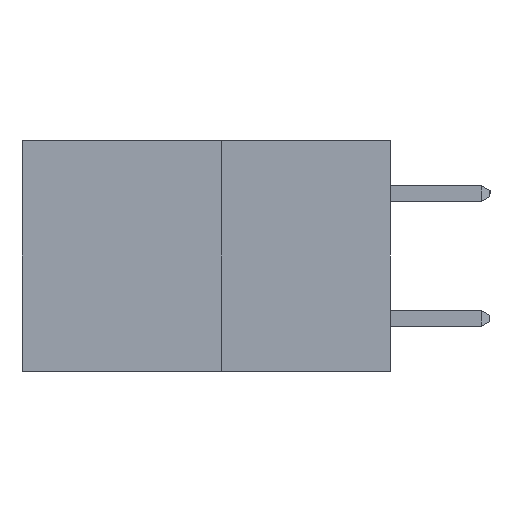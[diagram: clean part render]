
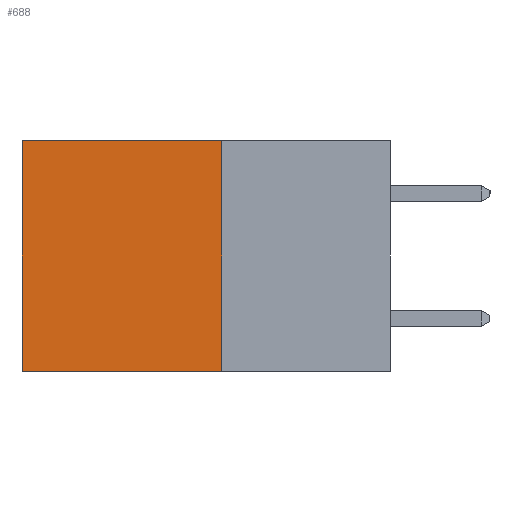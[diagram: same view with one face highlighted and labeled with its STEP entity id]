
A CAD part, left-side view. The second image highlights one B-rep face of the part: STEP entity #688.
In plain terms, the highlighted planar face has unit normal (-1, 0, 0).
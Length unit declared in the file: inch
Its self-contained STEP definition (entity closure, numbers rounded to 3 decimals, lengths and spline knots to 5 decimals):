
#74 = EDGE_CURVE ( 'NONE', #7495, #535, #5018, .T. ) ;
#273 = EDGE_LOOP ( 'NONE', ( #4200, #5590, #5253, #2440 ) ) ;
#535 = VERTEX_POINT ( 'NONE', #8804 ) ;
#688 = ADVANCED_FACE ( 'NONE', ( #9331 ), #6333, .F. ) ;
#1500 = DIRECTION ( 'NONE',  ( 1., 0., 0. ) ) ;
#1532 = VECTOR ( 'NONE', #4973, 39.37008 ) ;
#1788 = DIRECTION ( 'NONE',  ( 0., 1., 0. ) ) ;
#2301 = LINE ( 'NONE', #4025, #3783 ) ;
#2440 = ORIENTED_EDGE ( 'NONE', *, *, #3408, .T. ) ;
#2899 = VERTEX_POINT ( 'NONE', #4318 ) ;
#3270 = DIRECTION ( 'NONE',  ( 0., 0., -1. ) ) ;
#3338 = CARTESIAN_POINT ( 'NONE',  ( 0.277, 0.27, -0.37 ) ) ;
#3408 = EDGE_CURVE ( 'NONE', #4252, #2899, #2301, .T. ) ;
#3503 = LINE ( 'NONE', #4363, #1532 ) ;
#3783 = VECTOR ( 'NONE', #7253, 39.37008 ) ;
#3998 = CARTESIAN_POINT ( 'NONE',  ( 0.277, 0.27, 0. ) ) ;
#4025 = CARTESIAN_POINT ( 'NONE',  ( 0.277, 0.27, 0. ) ) ;
#4200 = ORIENTED_EDGE ( 'NONE', *, *, #6737, .T. ) ;
#4252 = VERTEX_POINT ( 'NONE', #3998 ) ;
#4318 = CARTESIAN_POINT ( 'NONE',  ( 0.277, 0.59, 0. ) ) ;
#4363 = CARTESIAN_POINT ( 'NONE',  ( 0.277, 0.59, -0.37 ) ) ;
#4973 = DIRECTION ( 'NONE',  ( 0., 0., -1. ) ) ;
#5018 = LINE ( 'NONE', #9354, #8589 ) ;
#5253 = ORIENTED_EDGE ( 'NONE', *, *, #5962, .F. ) ;
#5322 = CARTESIAN_POINT ( 'NONE',  ( 0.277, 0.27, -0.37 ) ) ;
#5590 = ORIENTED_EDGE ( 'NONE', *, *, #74, .F. ) ;
#5595 = DIRECTION ( 'NONE',  ( 0., 0., -1. ) ) ;
#5962 = EDGE_CURVE ( 'NONE', #4252, #7495, #8207, .T. ) ;
#6333 = PLANE ( 'NONE',  #7731 ) ;
#6360 = VECTOR ( 'NONE', #3270, 39.37008 ) ;
#6737 = EDGE_CURVE ( 'NONE', #2899, #535, #3503, .T. ) ;
#7253 = DIRECTION ( 'NONE',  ( 0., 1., 0. ) ) ;
#7495 = VERTEX_POINT ( 'NONE', #5322 ) ;
#7731 = AXIS2_PLACEMENT_3D ( 'NONE', #8339, #1500, #5595 ) ;
#8207 = LINE ( 'NONE', #3338, #6360 ) ;
#8339 = CARTESIAN_POINT ( 'NONE',  ( 0.277, 0.27, -0.37 ) ) ;
#8589 = VECTOR ( 'NONE', #1788, 39.37008 ) ;
#8804 = CARTESIAN_POINT ( 'NONE',  ( 0.277, 0.59, -0.37 ) ) ;
#9331 = FACE_OUTER_BOUND ( 'NONE', #273, .T. ) ;
#9354 = CARTESIAN_POINT ( 'NONE',  ( 0.277, 0.27, -0.37 ) ) ;
